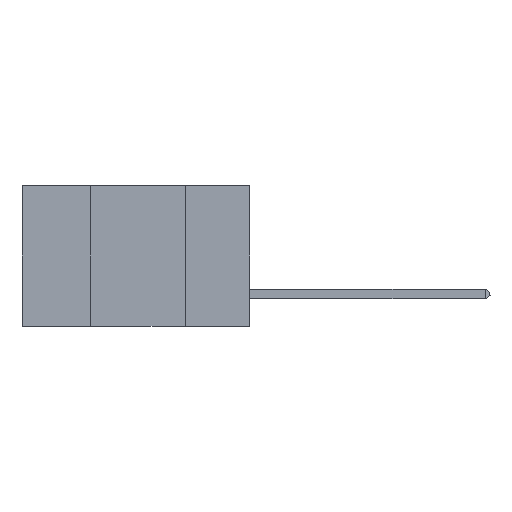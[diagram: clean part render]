
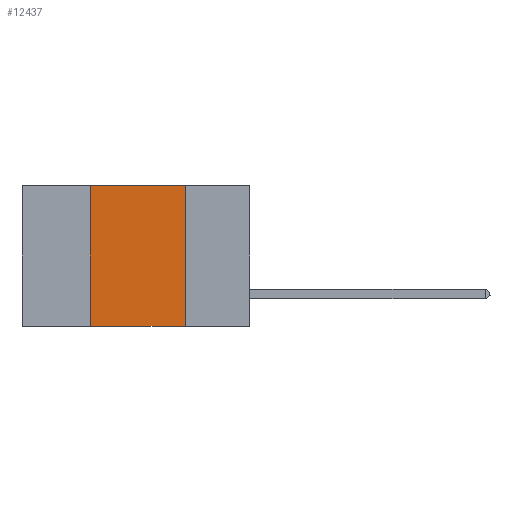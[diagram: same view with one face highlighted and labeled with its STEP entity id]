
A CAD part, left-side view. The second image highlights one B-rep face of the part: STEP entity #12437.
In plain terms, the highlighted planar face has unit normal (-1, 0, 0).
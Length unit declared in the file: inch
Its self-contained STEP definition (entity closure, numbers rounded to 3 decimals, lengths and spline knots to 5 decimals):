
#42 = PLANE ( 'NONE',  #5605 ) ;
#105 = VERTEX_POINT ( 'NONE', #13920 ) ;
#1254 = DIRECTION ( 'NONE',  ( 1., 0., 0. ) ) ;
#1598 = FACE_OUTER_BOUND ( 'NONE', #10642, .T. ) ;
#1757 = EDGE_CURVE ( 'NONE', #10230, #9452, #8169, .T. ) ;
#2129 = ORIENTED_EDGE ( 'NONE', *, *, #8039, .F. ) ;
#2192 = CARTESIAN_POINT ( 'NONE',  ( 0., 0.42, 0. ) ) ;
#2557 = CARTESIAN_POINT ( 'NONE',  ( 0., 0.6, -0.37 ) ) ;
#3789 = DIRECTION ( 'NONE',  ( 0., -1., 0. ) ) ;
#4057 = LINE ( 'NONE', #2557, #9878 ) ;
#4781 = DIRECTION ( 'NONE',  ( 0., 0., -1. ) ) ;
#4940 = DIRECTION ( 'NONE',  ( 0., -1., 0. ) ) ;
#5348 = EDGE_CURVE ( 'NONE', #10230, #105, #4057, .T. ) ;
#5605 = AXIS2_PLACEMENT_3D ( 'NONE', #8206, #1254, #4781 ) ;
#5665 = EDGE_CURVE ( 'NONE', #9452, #9605, #10596, .T. ) ;
#5904 = CARTESIAN_POINT ( 'NONE',  ( 0., 0.17, 0. ) ) ;
#6071 = ORIENTED_EDGE ( 'NONE', *, *, #5348, .T. ) ;
#6205 = VECTOR ( 'NONE', #13434, 39.37008 ) ;
#6600 = CARTESIAN_POINT ( 'NONE',  ( 0., 0.6, 0. ) ) ;
#7523 = VECTOR ( 'NONE', #3789, 39.37008 ) ;
#8039 = EDGE_CURVE ( 'NONE', #9605, #105, #11634, .T. ) ;
#8169 = LINE ( 'NONE', #10106, #11426 ) ;
#8206 = CARTESIAN_POINT ( 'NONE',  ( 0., 0.6, 0. ) ) ;
#9452 = VERTEX_POINT ( 'NONE', #2192 ) ;
#9605 = VERTEX_POINT ( 'NONE', #5904 ) ;
#9878 = VECTOR ( 'NONE', #4940, 39.37008 ) ;
#10106 = CARTESIAN_POINT ( 'NONE',  ( 0., 0.42, 0. ) ) ;
#10230 = VERTEX_POINT ( 'NONE', #11163 ) ;
#10596 = LINE ( 'NONE', #6600, #7523 ) ;
#10642 = EDGE_LOOP ( 'NONE', ( #2129, #11324, #14769, #6071 ) ) ;
#11163 = CARTESIAN_POINT ( 'NONE',  ( 0., 0.42, -0.37 ) ) ;
#11324 = ORIENTED_EDGE ( 'NONE', *, *, #5665, .F. ) ;
#11426 = VECTOR ( 'NONE', #12450, 39.37008 ) ;
#11634 = LINE ( 'NONE', #12284, #6205 ) ;
#12284 = CARTESIAN_POINT ( 'NONE',  ( 0., 0.17, 0. ) ) ;
#12437 = ADVANCED_FACE ( 'NONE', ( #1598 ), #42, .F. ) ;
#12450 = DIRECTION ( 'NONE',  ( 0., 0., 1. ) ) ;
#13434 = DIRECTION ( 'NONE',  ( 0., 0., -1. ) ) ;
#13920 = CARTESIAN_POINT ( 'NONE',  ( 0., 0.17, -0.37 ) ) ;
#14769 = ORIENTED_EDGE ( 'NONE', *, *, #1757, .F. ) ;
